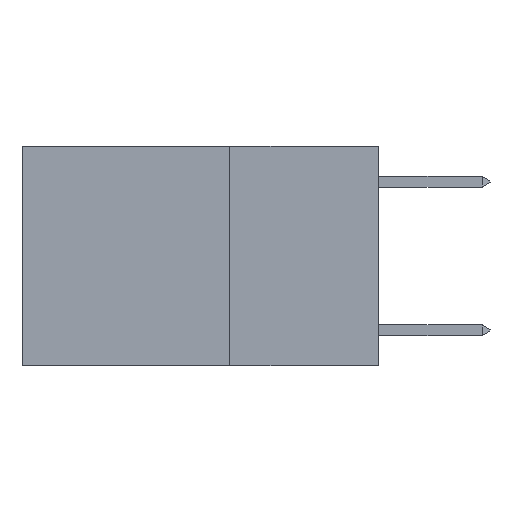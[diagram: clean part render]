
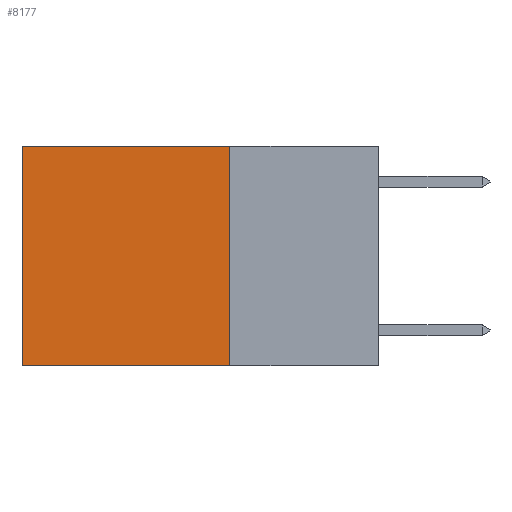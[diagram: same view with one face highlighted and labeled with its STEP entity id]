
A CAD part, left-side view. The second image highlights one B-rep face of the part: STEP entity #8177.
In plain terms, the highlighted planar face has unit normal (-1, 0, 0).
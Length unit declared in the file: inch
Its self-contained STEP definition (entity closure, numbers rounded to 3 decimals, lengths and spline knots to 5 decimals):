
#92 = CARTESIAN_POINT ( 'NONE',  ( 0.2625, 0.6, 0. ) ) ;
#164 = EDGE_LOOP ( 'NONE', ( #7266, #8835, #12900, #13078 ) ) ;
#1165 = CARTESIAN_POINT ( 'NONE',  ( 0.2625, 0.25, 0. ) ) ;
#1259 = PLANE ( 'NONE',  #9786 ) ;
#2031 = VERTEX_POINT ( 'NONE', #11895 ) ;
#2680 = VECTOR ( 'NONE', #3209, 39.37008 ) ;
#2761 = VECTOR ( 'NONE', #4067, 39.37008 ) ;
#2976 = LINE ( 'NONE', #8287, #2761 ) ;
#3209 = DIRECTION ( 'NONE',  ( 0., 0., -1. ) ) ;
#4067 = DIRECTION ( 'NONE',  ( 0., 1., 0. ) ) ;
#4767 = DIRECTION ( 'NONE',  ( 0., 1., 0. ) ) ;
#5027 = VECTOR ( 'NONE', #10761, 39.37008 ) ;
#5797 = EDGE_CURVE ( 'NONE', #2031, #8428, #12898, .T. ) ;
#5907 = CARTESIAN_POINT ( 'NONE',  ( 0.2625, 0.6, -0.37 ) ) ;
#6750 = CARTESIAN_POINT ( 'NONE',  ( 0.2625, 0.25, -0.37 ) ) ;
#7081 = VERTEX_POINT ( 'NONE', #1165 ) ;
#7266 = ORIENTED_EDGE ( 'NONE', *, *, #5797, .T. ) ;
#7442 = VERTEX_POINT ( 'NONE', #9004 ) ;
#7445 = EDGE_CURVE ( 'NONE', #7442, #8428, #13247, .T. ) ;
#7488 = CARTESIAN_POINT ( 'NONE',  ( 0.2625, 0.25, 0. ) ) ;
#7657 = EDGE_CURVE ( 'NONE', #7081, #7442, #8336, .T. ) ;
#7676 = FACE_OUTER_BOUND ( 'NONE', #164, .T. ) ;
#7740 = CARTESIAN_POINT ( 'NONE',  ( 0.2625, 0.25, 0. ) ) ;
#8177 = ADVANCED_FACE ( 'NONE', ( #7676 ), #1259, .F. ) ;
#8287 = CARTESIAN_POINT ( 'NONE',  ( 0.2625, 0.25, 0. ) ) ;
#8336 = LINE ( 'NONE', #7488, #5027 ) ;
#8428 = VERTEX_POINT ( 'NONE', #5907 ) ;
#8814 = DIRECTION ( 'NONE',  ( 1., 0., 0. ) ) ;
#8835 = ORIENTED_EDGE ( 'NONE', *, *, #7445, .F. ) ;
#9004 = CARTESIAN_POINT ( 'NONE',  ( 0.2625, 0.25, -0.37 ) ) ;
#9786 = AXIS2_PLACEMENT_3D ( 'NONE', #7740, #8814, #13121 ) ;
#10269 = EDGE_CURVE ( 'NONE', #7081, #2031, #2976, .T. ) ;
#10761 = DIRECTION ( 'NONE',  ( 0., 0., -1. ) ) ;
#11895 = CARTESIAN_POINT ( 'NONE',  ( 0.2625, 0.6, 0. ) ) ;
#12898 = LINE ( 'NONE', #92, #2680 ) ;
#12900 = ORIENTED_EDGE ( 'NONE', *, *, #7657, .F. ) ;
#13078 = ORIENTED_EDGE ( 'NONE', *, *, #10269, .T. ) ;
#13121 = DIRECTION ( 'NONE',  ( 0., 0., -1. ) ) ;
#13247 = LINE ( 'NONE', #6750, #13591 ) ;
#13591 = VECTOR ( 'NONE', #4767, 39.37008 ) ;
